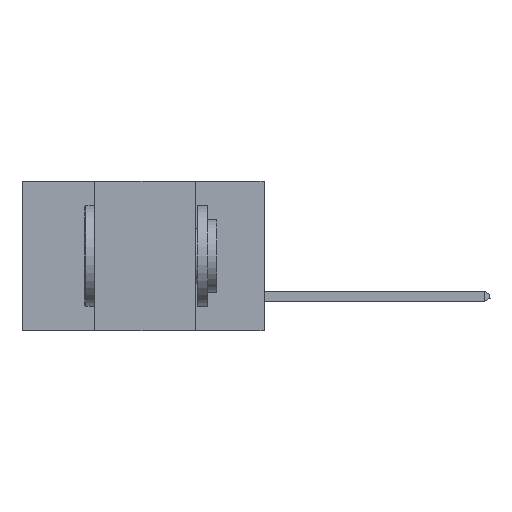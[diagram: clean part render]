
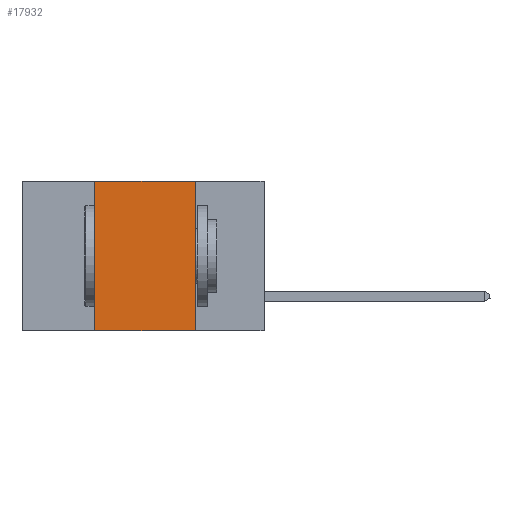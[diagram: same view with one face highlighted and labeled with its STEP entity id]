
A CAD part, left-side view. The second image highlights one B-rep face of the part: STEP entity #17932.
In plain terms, the highlighted planar face has unit normal (-1, 0, 0).
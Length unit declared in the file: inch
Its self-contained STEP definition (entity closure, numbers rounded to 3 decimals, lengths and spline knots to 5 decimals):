
#358 = EDGE_CURVE ( 'NONE', #8566, #11985, #1008, .T. ) ;
#1008 = LINE ( 'NONE', #3735, #10370 ) ;
#1353 = DIRECTION ( 'NONE',  ( 1., 0., 0. ) ) ;
#1542 = CARTESIAN_POINT ( 'NONE',  ( 0., 0.17, 0. ) ) ;
#3158 = FACE_OUTER_BOUND ( 'NONE', #3894, .T. ) ;
#3187 = CARTESIAN_POINT ( 'NONE',  ( 0., 0.17, -0.37 ) ) ;
#3188 = DIRECTION ( 'NONE',  ( 0., 0., -1. ) ) ;
#3215 = EDGE_CURVE ( 'NONE', #8566, #20430, #7881, .T. ) ;
#3735 = CARTESIAN_POINT ( 'NONE',  ( 0., 0.42, 0. ) ) ;
#3894 = EDGE_LOOP ( 'NONE', ( #20549, #6024, #17470, #20181 ) ) ;
#3964 = DIRECTION ( 'NONE',  ( 0., 0., 1. ) ) ;
#4472 = CARTESIAN_POINT ( 'NONE',  ( 0., 0.6, 0. ) ) ;
#5314 = LINE ( 'NONE', #12138, #16340 ) ;
#5422 = LINE ( 'NONE', #1542, #9344 ) ;
#5697 = EDGE_CURVE ( 'NONE', #7242, #20430, #5422, .T. ) ;
#6024 = ORIENTED_EDGE ( 'NONE', *, *, #16265, .F. ) ;
#7242 = VERTEX_POINT ( 'NONE', #9340 ) ;
#7881 = LINE ( 'NONE', #18614, #12329 ) ;
#8378 = CARTESIAN_POINT ( 'NONE',  ( 0., 0.42, 0. ) ) ;
#8566 = VERTEX_POINT ( 'NONE', #9903 ) ;
#8636 = DIRECTION ( 'NONE',  ( 0., -1., 0. ) ) ;
#9340 = CARTESIAN_POINT ( 'NONE',  ( 0., 0.17, 0. ) ) ;
#9344 = VECTOR ( 'NONE', #3188, 39.37008 ) ;
#9903 = CARTESIAN_POINT ( 'NONE',  ( 0., 0.42, -0.37 ) ) ;
#10370 = VECTOR ( 'NONE', #3964, 39.37008 ) ;
#11985 = VERTEX_POINT ( 'NONE', #8378 ) ;
#12138 = CARTESIAN_POINT ( 'NONE',  ( 0., 0.6, 0. ) ) ;
#12329 = VECTOR ( 'NONE', #8636, 39.37008 ) ;
#13843 = DIRECTION ( 'NONE',  ( 0., -1., 0. ) ) ;
#14630 = PLANE ( 'NONE',  #18298 ) ;
#16265 = EDGE_CURVE ( 'NONE', #11985, #7242, #5314, .T. ) ;
#16340 = VECTOR ( 'NONE', #13843, 39.37008 ) ;
#17470 = ORIENTED_EDGE ( 'NONE', *, *, #358, .F. ) ;
#17932 = ADVANCED_FACE ( 'NONE', ( #3158 ), #14630, .F. ) ;
#18016 = DIRECTION ( 'NONE',  ( 0., 0., -1. ) ) ;
#18298 = AXIS2_PLACEMENT_3D ( 'NONE', #4472, #1353, #18016 ) ;
#18614 = CARTESIAN_POINT ( 'NONE',  ( 0., 0.6, -0.37 ) ) ;
#20181 = ORIENTED_EDGE ( 'NONE', *, *, #3215, .T. ) ;
#20430 = VERTEX_POINT ( 'NONE', #3187 ) ;
#20549 = ORIENTED_EDGE ( 'NONE', *, *, #5697, .F. ) ;
